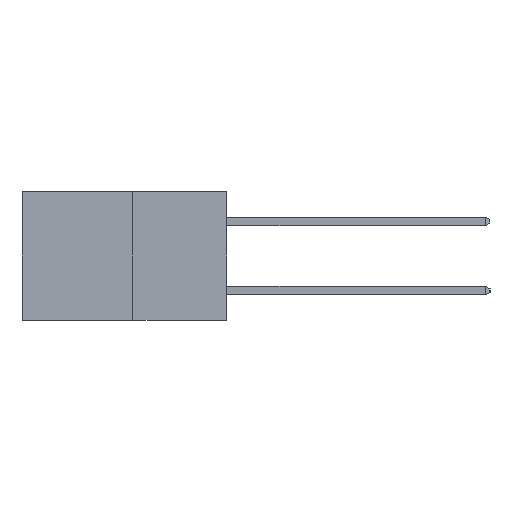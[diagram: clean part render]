
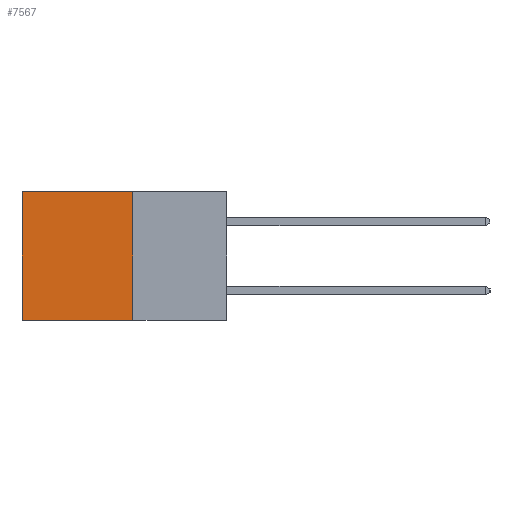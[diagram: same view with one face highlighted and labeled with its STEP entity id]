
A CAD part, left-side view. The second image highlights one B-rep face of the part: STEP entity #7567.
In plain terms, the highlighted planar face has unit normal (-1, 0, 0).
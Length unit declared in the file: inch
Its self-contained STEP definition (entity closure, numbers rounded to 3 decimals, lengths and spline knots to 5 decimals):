
#135 = DIRECTION ( 'NONE',  ( 0., 1., 0. ) ) ;
#587 = PLANE ( 'NONE',  #6259 ) ;
#670 = VERTEX_POINT ( 'NONE', #3715 ) ;
#1008 = LINE ( 'NONE', #2175, #6579 ) ;
#1352 = CARTESIAN_POINT ( 'NONE',  ( 0.277, 0.27, -0.37 ) ) ;
#1486 = VECTOR ( 'NONE', #6426, 39.37008 ) ;
#1699 = EDGE_CURVE ( 'NONE', #670, #7005, #1991, .T. ) ;
#1933 = VERTEX_POINT ( 'NONE', #6602 ) ;
#1991 = LINE ( 'NONE', #7230, #9900 ) ;
#2128 = DIRECTION ( 'NONE',  ( 0., 0., -1. ) ) ;
#2175 = CARTESIAN_POINT ( 'NONE',  ( 0.277, 0.59, -0.37 ) ) ;
#2643 = EDGE_LOOP ( 'NONE', ( #5907, #6655, #8211, #9773 ) ) ;
#2846 = CARTESIAN_POINT ( 'NONE',  ( 0.277, 0.59, -0.37 ) ) ;
#2971 = VERTEX_POINT ( 'NONE', #6716 ) ;
#3496 = LINE ( 'NONE', #4127, #1486 ) ;
#3715 = CARTESIAN_POINT ( 'NONE',  ( 0.277, 0.27, -0.37 ) ) ;
#4127 = CARTESIAN_POINT ( 'NONE',  ( 0.277, 0.27, -0.37 ) ) ;
#5907 = ORIENTED_EDGE ( 'NONE', *, *, #8903, .T. ) ;
#6259 = AXIS2_PLACEMENT_3D ( 'NONE', #1352, #6656, #2128 ) ;
#6426 = DIRECTION ( 'NONE',  ( 0., 0., -1. ) ) ;
#6579 = VECTOR ( 'NONE', #6715, 39.37008 ) ;
#6602 = CARTESIAN_POINT ( 'NONE',  ( 0.277, 0.59, 0. ) ) ;
#6655 = ORIENTED_EDGE ( 'NONE', *, *, #1699, .F. ) ;
#6656 = DIRECTION ( 'NONE',  ( 1., 0., 0. ) ) ;
#6715 = DIRECTION ( 'NONE',  ( 0., 0., -1. ) ) ;
#6716 = CARTESIAN_POINT ( 'NONE',  ( 0.277, 0.27, 0. ) ) ;
#7005 = VERTEX_POINT ( 'NONE', #2846 ) ;
#7230 = CARTESIAN_POINT ( 'NONE',  ( 0.277, 0.27, -0.37 ) ) ;
#7385 = EDGE_CURVE ( 'NONE', #2971, #1933, #9884, .T. ) ;
#7395 = EDGE_CURVE ( 'NONE', #2971, #670, #3496, .T. ) ;
#7545 = VECTOR ( 'NONE', #8734, 39.37008 ) ;
#7567 = ADVANCED_FACE ( 'NONE', ( #7934 ), #587, .F. ) ;
#7934 = FACE_OUTER_BOUND ( 'NONE', #2643, .T. ) ;
#8211 = ORIENTED_EDGE ( 'NONE', *, *, #7395, .F. ) ;
#8734 = DIRECTION ( 'NONE',  ( 0., 1., 0. ) ) ;
#8903 = EDGE_CURVE ( 'NONE', #1933, #7005, #1008, .T. ) ;
#9538 = CARTESIAN_POINT ( 'NONE',  ( 0.277, 0.27, 0. ) ) ;
#9773 = ORIENTED_EDGE ( 'NONE', *, *, #7385, .T. ) ;
#9884 = LINE ( 'NONE', #9538, #7545 ) ;
#9900 = VECTOR ( 'NONE', #135, 39.37008 ) ;
